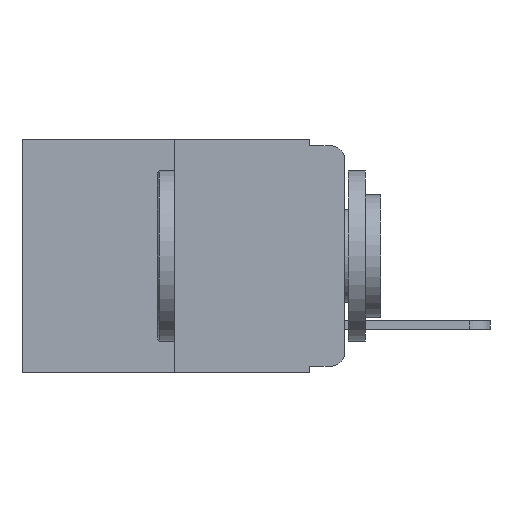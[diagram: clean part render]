
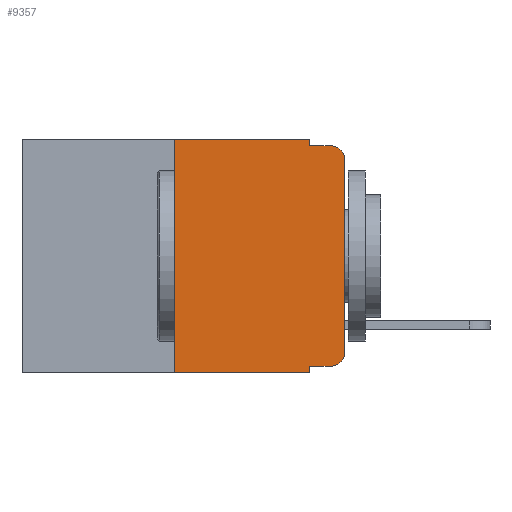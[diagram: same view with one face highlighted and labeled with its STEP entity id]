
A CAD part, left-side view. The second image highlights one B-rep face of the part: STEP entity #9357.
In plain terms, the highlighted planar face has unit normal (-1, 0, 0).
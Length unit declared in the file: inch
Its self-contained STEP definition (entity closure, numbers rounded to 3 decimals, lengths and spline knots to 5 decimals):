
#457 = CARTESIAN_POINT ( 'NONE',  ( 0., 0.051, -0.333 ) ) ;
#539 = VERTEX_POINT ( 'NONE', #2482 ) ;
#573 = CARTESIAN_POINT ( 'NONE',  ( 0., 0.02, -0.01 ) ) ;
#1347 = VERTEX_POINT ( 'NONE', #8381 ) ;
#1450 = VERTEX_POINT ( 'NONE', #7280 ) ;
#1693 = EDGE_CURVE ( 'NONE', #7484, #2904, #6540, .T. ) ;
#2065 = CARTESIAN_POINT ( 'NONE',  ( 0., 0.02, -0.333 ) ) ;
#2384 = LINE ( 'NONE', #12521, #8017 ) ;
#2406 = CARTESIAN_POINT ( 'NONE',  ( 0., 0., -0.03 ) ) ;
#2482 = CARTESIAN_POINT ( 'NONE',  ( 0., 0.051, -0.333 ) ) ;
#2568 = LINE ( 'NONE', #10376, #12725 ) ;
#2601 = DIRECTION ( 'NONE',  ( 0., -1., 0. ) ) ;
#2803 = DIRECTION ( 'NONE',  ( 0., 0., -1. ) ) ;
#2816 = CARTESIAN_POINT ( 'NONE',  ( 0., 0.051, 0. ) ) ;
#2839 = AXIS2_PLACEMENT_3D ( 'NONE', #10075, #9636, #9490 ) ;
#2904 = VERTEX_POINT ( 'NONE', #10114 ) ;
#2968 = VERTEX_POINT ( 'NONE', #573 ) ;
#3136 = EDGE_CURVE ( 'NONE', #6981, #9787, #7097, .T. ) ;
#3289 = VECTOR ( 'NONE', #8853, 39.37008 ) ;
#3474 = EDGE_CURVE ( 'NONE', #8756, #2968, #5389, .T. ) ;
#3921 = DIRECTION ( 'NONE',  ( 0., -1., 0. ) ) ;
#4186 = LINE ( 'NONE', #11241, #3289 ) ;
#4256 = ORIENTED_EDGE ( 'NONE', *, *, #12740, .T. ) ;
#4314 = ORIENTED_EDGE ( 'NONE', *, *, #3474, .T. ) ;
#4407 = ORIENTED_EDGE ( 'NONE', *, *, #13020, .F. ) ;
#4435 = ORIENTED_EDGE ( 'NONE', *, *, #11099, .F. ) ;
#4540 = ORIENTED_EDGE ( 'NONE', *, *, #6679, .F. ) ;
#4553 = DIRECTION ( 'NONE',  ( 0., 0., -1. ) ) ;
#4564 = LINE ( 'NONE', #6153, #9844 ) ;
#4695 = ORIENTED_EDGE ( 'NONE', *, *, #7597, .F. ) ;
#4712 = CARTESIAN_POINT ( 'NONE',  ( 0., 0.051, -0.01 ) ) ;
#4768 = ORIENTED_EDGE ( 'NONE', *, *, #3136, .T. ) ;
#4857 = LINE ( 'NONE', #457, #12902 ) ;
#4914 = DIRECTION ( 'NONE',  ( -1., 0., 0. ) ) ;
#4923 = CARTESIAN_POINT ( 'NONE',  ( 0., 0.02, -0.03 ) ) ;
#4940 = ORIENTED_EDGE ( 'NONE', *, *, #7958, .F. ) ;
#4966 = ORIENTED_EDGE ( 'NONE', *, *, #7957, .T. ) ;
#5190 = DIRECTION ( 'NONE',  ( 0., -1., 0. ) ) ;
#5207 = DIRECTION ( 'NONE',  ( 0., 0., -1. ) ) ;
#5208 = ORIENTED_EDGE ( 'NONE', *, *, #1693, .T. ) ;
#5209 = DIRECTION ( 'NONE',  ( -1., 0., 0. ) ) ;
#5222 = CARTESIAN_POINT ( 'NONE',  ( 0., 0.02, -0.313 ) ) ;
#5389 = CIRCLE ( 'NONE', #11878, 0.02 ) ;
#5923 = CARTESIAN_POINT ( 'NONE',  ( 0., 0.473, -0.343 ) ) ;
#6153 = CARTESIAN_POINT ( 'NONE',  ( 0., 0.051, 0. ) ) ;
#6540 = CIRCLE ( 'NONE', #12978, 0.02 ) ;
#6679 = EDGE_CURVE ( 'NONE', #1450, #1347, #4186, .T. ) ;
#6778 = LINE ( 'NONE', #2816, #12150 ) ;
#6981 = VERTEX_POINT ( 'NONE', #9182 ) ;
#7097 = LINE ( 'NONE', #5923, #7532 ) ;
#7171 = DIRECTION ( 'NONE',  ( 0., 0., -1. ) ) ;
#7280 = CARTESIAN_POINT ( 'NONE',  ( 0., 0.25, 0. ) ) ;
#7430 = VERTEX_POINT ( 'NONE', #4712 ) ;
#7484 = VERTEX_POINT ( 'NONE', #2065 ) ;
#7532 = VECTOR ( 'NONE', #2601, 39.37008 ) ;
#7545 = DIRECTION ( 'NONE',  ( 0., 0., 1. ) ) ;
#7597 = EDGE_CURVE ( 'NONE', #6981, #1450, #10501, .T. ) ;
#7656 = CARTESIAN_POINT ( 'NONE',  ( 0., 0.25, 0. ) ) ;
#7957 = EDGE_CURVE ( 'NONE', #539, #7484, #4857, .T. ) ;
#7958 = EDGE_CURVE ( 'NONE', #539, #9787, #4564, .T. ) ;
#8017 = VECTOR ( 'NONE', #8077, 39.37008 ) ;
#8077 = DIRECTION ( 'NONE',  ( 0., 0., 1. ) ) ;
#8381 = CARTESIAN_POINT ( 'NONE',  ( 0., 0.051, 0. ) ) ;
#8756 = VERTEX_POINT ( 'NONE', #2406 ) ;
#8853 = DIRECTION ( 'NONE',  ( 0., -1., 0. ) ) ;
#9182 = CARTESIAN_POINT ( 'NONE',  ( 0., 0.25, -0.343 ) ) ;
#9357 = ADVANCED_FACE ( 'NONE', ( #11340 ), #10371, .F. ) ;
#9490 = DIRECTION ( 'NONE',  ( 0., 0., -1. ) ) ;
#9636 = DIRECTION ( 'NONE',  ( 1., 0., 0. ) ) ;
#9787 = VERTEX_POINT ( 'NONE', #10161 ) ;
#9844 = VECTOR ( 'NONE', #4553, 39.37008 ) ;
#10075 = CARTESIAN_POINT ( 'NONE',  ( 0., 0.473, 0. ) ) ;
#10114 = CARTESIAN_POINT ( 'NONE',  ( 0., 0., -0.313 ) ) ;
#10137 = EDGE_LOOP ( 'NONE', ( #4256, #4314, #4407, #4435, #4540, #4695, #4768, #4940, #4966, #5208 ) ) ;
#10161 = CARTESIAN_POINT ( 'NONE',  ( 0., 0.051, -0.343 ) ) ;
#10371 = PLANE ( 'NONE',  #2839 ) ;
#10376 = CARTESIAN_POINT ( 'NONE',  ( 0., 0.051, -0.01 ) ) ;
#10501 = LINE ( 'NONE', #7656, #12394 ) ;
#11099 = EDGE_CURVE ( 'NONE', #1347, #7430, #6778, .T. ) ;
#11241 = CARTESIAN_POINT ( 'NONE',  ( 0., 0.473, 0. ) ) ;
#11340 = FACE_OUTER_BOUND ( 'NONE', #10137, .T. ) ;
#11878 = AXIS2_PLACEMENT_3D ( 'NONE', #4923, #4914, #7171 ) ;
#12150 = VECTOR ( 'NONE', #2803, 39.37008 ) ;
#12394 = VECTOR ( 'NONE', #7545, 39.37008 ) ;
#12521 = CARTESIAN_POINT ( 'NONE',  ( 0., 0., 0. ) ) ;
#12725 = VECTOR ( 'NONE', #5190, 39.37008 ) ;
#12740 = EDGE_CURVE ( 'NONE', #2904, #8756, #2384, .T. ) ;
#12902 = VECTOR ( 'NONE', #3921, 39.37008 ) ;
#12978 = AXIS2_PLACEMENT_3D ( 'NONE', #5222, #5209, #5207 ) ;
#13020 = EDGE_CURVE ( 'NONE', #7430, #2968, #2568, .T. ) ;
